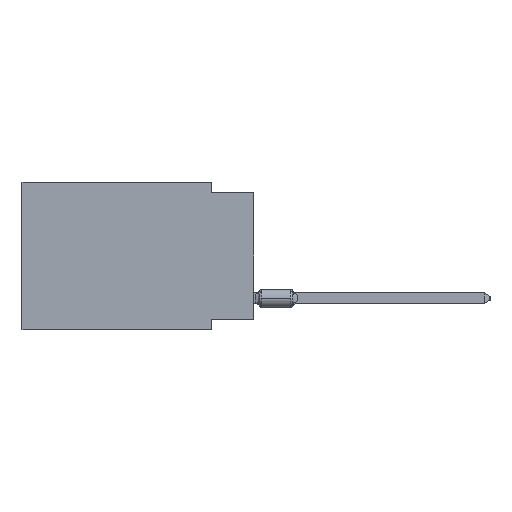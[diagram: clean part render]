
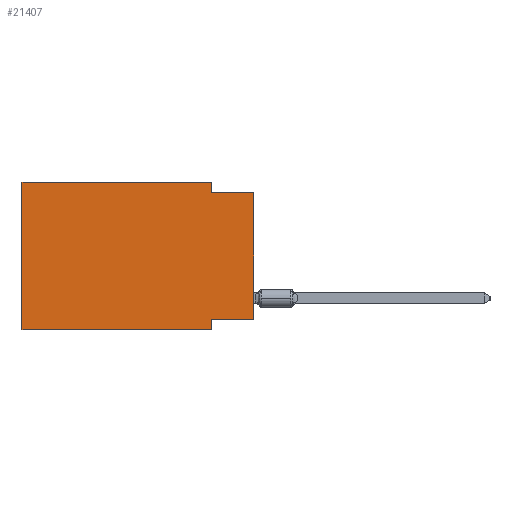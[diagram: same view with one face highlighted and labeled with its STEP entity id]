
A CAD part, left-side view. The second image highlights one B-rep face of the part: STEP entity #21407.
In plain terms, the highlighted planar face has unit normal (-1, 0, 0).
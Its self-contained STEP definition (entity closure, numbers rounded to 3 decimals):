
#1299 = CARTESIAN_POINT ( 'NONE',  ( 0., 13.97, -8.89 ) ) ;
#3568 = CARTESIAN_POINT ( 'NONE',  ( 0., 0., -8.255 ) ) ;
#4810 = FACE_OUTER_BOUND ( 'NONE', #42308, .T. ) ;
#6616 = VERTEX_POINT ( 'NONE', #3568 ) ;
#7075 = EDGE_CURVE ( 'NONE', #68864, #51417, #51618, .T. ) ;
#8008 = LINE ( 'NONE', #73828, #19169 ) ;
#10021 = CARTESIAN_POINT ( 'NONE',  ( 0., 2.54, 0. ) ) ;
#10343 = LINE ( 'NONE', #26066, #67106 ) ;
#12483 = VECTOR ( 'NONE', #50220, 1000. ) ;
#13761 = DIRECTION ( 'NONE',  ( 0., 0., 1. ) ) ;
#13864 = VECTOR ( 'NONE', #17433, 1000. ) ;
#13872 = DIRECTION ( 'NONE',  ( 0., 0., -1. ) ) ;
#15994 = CARTESIAN_POINT ( 'NONE',  ( 0., 0., -0.635 ) ) ;
#16698 = EDGE_CURVE ( 'NONE', #51417, #57645, #47933, .T. ) ;
#17120 = PLANE ( 'NONE',  #36070 ) ;
#17433 = DIRECTION ( 'NONE',  ( 0., -1., 0. ) ) ;
#19169 = VECTOR ( 'NONE', #75385, 1000. ) ;
#19321 = ORIENTED_EDGE ( 'NONE', *, *, #30958, .T. ) ;
#19558 = CARTESIAN_POINT ( 'NONE',  ( 0., 2.54, -8.255 ) ) ;
#20049 = ORIENTED_EDGE ( 'NONE', *, *, #50734, .F. ) ;
#21407 = ADVANCED_FACE ( 'NONE', ( #4810 ), #17120, .F. ) ;
#21901 = CARTESIAN_POINT ( 'NONE',  ( 0., 13.97, 0. ) ) ;
#26066 = CARTESIAN_POINT ( 'NONE',  ( 0., 0., 0. ) ) ;
#26987 = EDGE_CURVE ( 'NONE', #60477, #30992, #39595, .T. ) ;
#27003 = DIRECTION ( 'NONE',  ( 0., 1., 0. ) ) ;
#29007 = CARTESIAN_POINT ( 'NONE',  ( 0., 13.97, 0. ) ) ;
#29196 = EDGE_CURVE ( 'NONE', #6616, #74900, #10343, .T. ) ;
#29710 = CARTESIAN_POINT ( 'NONE',  ( 0., 13.97, 0. ) ) ;
#29728 = CARTESIAN_POINT ( 'NONE',  ( 0., 0., -0.635 ) ) ;
#30958 = EDGE_CURVE ( 'NONE', #68864, #30992, #8008, .T. ) ;
#30992 = VERTEX_POINT ( 'NONE', #37340 ) ;
#32153 = CARTESIAN_POINT ( 'NONE',  ( 0., 0., -8.255 ) ) ;
#33913 = CARTESIAN_POINT ( 'NONE',  ( 0., 13.97, 0. ) ) ;
#34976 = DIRECTION ( 'NONE',  ( 0., 0., -1. ) ) ;
#36070 = AXIS2_PLACEMENT_3D ( 'NONE', #29007, #57932, #40886 ) ;
#37340 = CARTESIAN_POINT ( 'NONE',  ( 0., 2.54, -8.89 ) ) ;
#37809 = ORIENTED_EDGE ( 'NONE', *, *, #74800, .F. ) ;
#38112 = LINE ( 'NONE', #32153, #70137 ) ;
#39473 = ORIENTED_EDGE ( 'NONE', *, *, #16698, .F. ) ;
#39595 = LINE ( 'NONE', #68558, #77033 ) ;
#40272 = VECTOR ( 'NONE', #34976, 1000. ) ;
#40836 = VECTOR ( 'NONE', #76986, 1000. ) ;
#40886 = DIRECTION ( 'NONE',  ( 0., 0., -1. ) ) ;
#41313 = LINE ( 'NONE', #10021, #40272 ) ;
#42308 = EDGE_LOOP ( 'NONE', ( #43532, #65261, #20049, #39473, #64856, #19321, #63214, #37809 ) ) ;
#43532 = ORIENTED_EDGE ( 'NONE', *, *, #29196, .T. ) ;
#47933 = LINE ( 'NONE', #29710, #13864 ) ;
#49044 = CARTESIAN_POINT ( 'NONE',  ( 0., 2.54, 0. ) ) ;
#50220 = DIRECTION ( 'NONE',  ( 0., -1., 0. ) ) ;
#50734 = EDGE_CURVE ( 'NONE', #57645, #52991, #41313, .T. ) ;
#51417 = VERTEX_POINT ( 'NONE', #33913 ) ;
#51618 = LINE ( 'NONE', #21901, #40836 ) ;
#52991 = VERTEX_POINT ( 'NONE', #57040 ) ;
#57040 = CARTESIAN_POINT ( 'NONE',  ( 0., 2.54, -0.635 ) ) ;
#57645 = VERTEX_POINT ( 'NONE', #49044 ) ;
#57932 = DIRECTION ( 'NONE',  ( 1., 0., 0. ) ) ;
#58004 = LINE ( 'NONE', #15994, #12483 ) ;
#60477 = VERTEX_POINT ( 'NONE', #19558 ) ;
#63214 = ORIENTED_EDGE ( 'NONE', *, *, #26987, .F. ) ;
#64856 = ORIENTED_EDGE ( 'NONE', *, *, #7075, .F. ) ;
#65261 = ORIENTED_EDGE ( 'NONE', *, *, #65438, .F. ) ;
#65438 = EDGE_CURVE ( 'NONE', #52991, #74900, #58004, .T. ) ;
#67106 = VECTOR ( 'NONE', #13761, 1000. ) ;
#68558 = CARTESIAN_POINT ( 'NONE',  ( 0., 2.54, -8.89 ) ) ;
#68864 = VERTEX_POINT ( 'NONE', #1299 ) ;
#70137 = VECTOR ( 'NONE', #27003, 1000. ) ;
#73828 = CARTESIAN_POINT ( 'NONE',  ( 0., 13.97, -8.89 ) ) ;
#74800 = EDGE_CURVE ( 'NONE', #6616, #60477, #38112, .T. ) ;
#74900 = VERTEX_POINT ( 'NONE', #29728 ) ;
#75385 = DIRECTION ( 'NONE',  ( 0., -1., 0. ) ) ;
#76986 = DIRECTION ( 'NONE',  ( 0., 0., 1. ) ) ;
#77033 = VECTOR ( 'NONE', #13872, 1000. ) ;
